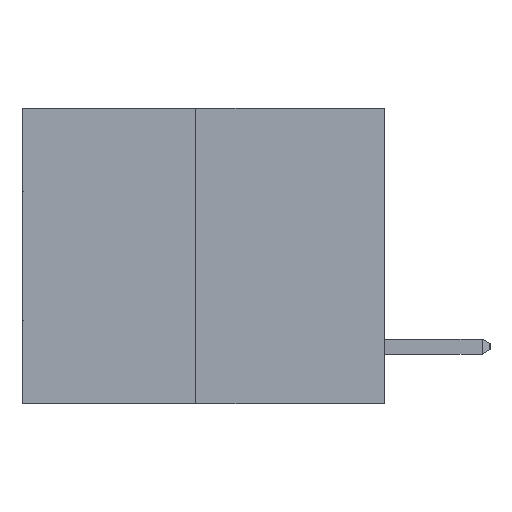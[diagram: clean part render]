
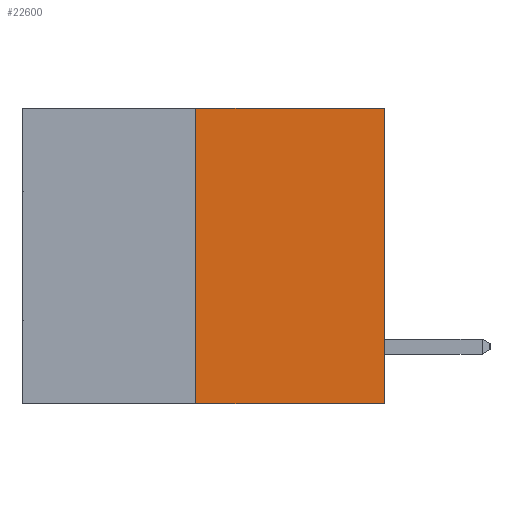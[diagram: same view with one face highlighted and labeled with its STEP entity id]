
A CAD part, left-side view. The second image highlights one B-rep face of the part: STEP entity #22600.
In plain terms, the highlighted planar face has unit normal (-1, 0, 0).
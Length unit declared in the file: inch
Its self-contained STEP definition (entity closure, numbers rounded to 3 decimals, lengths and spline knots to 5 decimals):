
#154 = ORIENTED_EDGE ( 'NONE', *, *, #24030, .F. ) ;
#831 = VECTOR ( 'NONE', #16812, 39.37008 ) ;
#1686 = CARTESIAN_POINT ( 'NONE',  ( 0., 0.6, 0. ) ) ;
#2529 = PLANE ( 'NONE',  #17787 ) ;
#3764 = VECTOR ( 'NONE', #24068, 39.37008 ) ;
#5383 = CARTESIAN_POINT ( 'NONE',  ( 0., 0.312, 0. ) ) ;
#6995 = CARTESIAN_POINT ( 'NONE',  ( 0., 0., -0.49 ) ) ;
#8866 = EDGE_LOOP ( 'NONE', ( #18460, #30677, #15996, #154 ) ) ;
#8874 = CARTESIAN_POINT ( 'NONE',  ( 0., 0.312, -0.49 ) ) ;
#11002 = CARTESIAN_POINT ( 'NONE',  ( 0., 0.6, -0.49 ) ) ;
#12393 = CARTESIAN_POINT ( 'NONE',  ( 0., 0.6, 0. ) ) ;
#12489 = DIRECTION ( 'NONE',  ( 0., 0., -1. ) ) ;
#13193 = VECTOR ( 'NONE', #26161, 39.37008 ) ;
#13305 = VERTEX_POINT ( 'NONE', #5383 ) ;
#13440 = DIRECTION ( 'NONE',  ( 0., -1., 0. ) ) ;
#14146 = EDGE_CURVE ( 'NONE', #24942, #15656, #19581, .T. ) ;
#15656 = VERTEX_POINT ( 'NONE', #6995 ) ;
#15996 = ORIENTED_EDGE ( 'NONE', *, *, #26760, .T. ) ;
#16812 = DIRECTION ( 'NONE',  ( 0., 0., 1. ) ) ;
#17425 = CARTESIAN_POINT ( 'NONE',  ( 0., 0., 0. ) ) ;
#17787 = AXIS2_PLACEMENT_3D ( 'NONE', #12393, #29478, #12489 ) ;
#18068 = VECTOR ( 'NONE', #13440, 39.37008 ) ;
#18330 = EDGE_CURVE ( 'NONE', #24942, #13305, #30038, .T. ) ;
#18460 = ORIENTED_EDGE ( 'NONE', *, *, #18330, .F. ) ;
#19581 = LINE ( 'NONE', #11002, #18068 ) ;
#20973 = LINE ( 'NONE', #1686, #3764 ) ;
#22287 = LINE ( 'NONE', #26622, #831 ) ;
#22600 = ADVANCED_FACE ( 'NONE', ( #27118 ), #2529, .F. ) ;
#24030 = EDGE_CURVE ( 'NONE', #13305, #29492, #20973, .T. ) ;
#24068 = DIRECTION ( 'NONE',  ( 0., -1., 0. ) ) ;
#24942 = VERTEX_POINT ( 'NONE', #8874 ) ;
#26161 = DIRECTION ( 'NONE',  ( 0., 0., 1. ) ) ;
#26371 = CARTESIAN_POINT ( 'NONE',  ( 0., 0.312, -0.49 ) ) ;
#26622 = CARTESIAN_POINT ( 'NONE',  ( 0., 0., 0. ) ) ;
#26760 = EDGE_CURVE ( 'NONE', #15656, #29492, #22287, .T. ) ;
#27118 = FACE_OUTER_BOUND ( 'NONE', #8866, .T. ) ;
#29478 = DIRECTION ( 'NONE',  ( 1., 0., 0. ) ) ;
#29492 = VERTEX_POINT ( 'NONE', #17425 ) ;
#30038 = LINE ( 'NONE', #26371, #13193 ) ;
#30677 = ORIENTED_EDGE ( 'NONE', *, *, #14146, .T. ) ;
